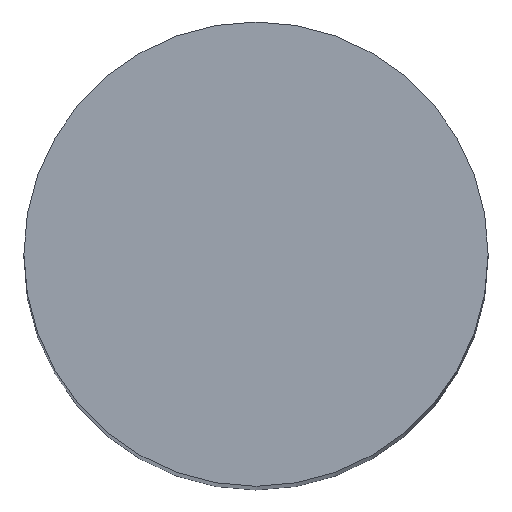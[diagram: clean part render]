
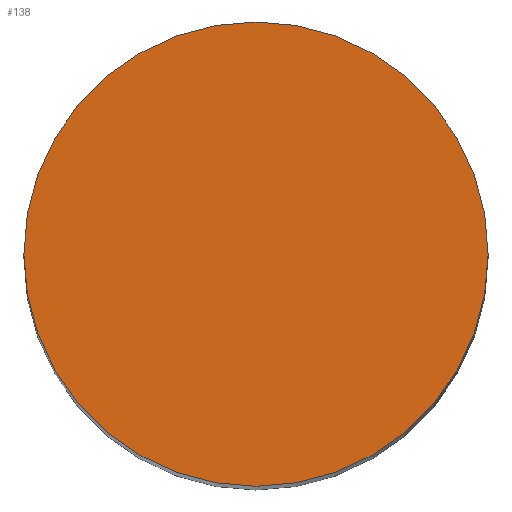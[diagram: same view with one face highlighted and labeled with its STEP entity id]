
A CAD part, top view. The second image highlights one B-rep face of the part: STEP entity #138.
In plain terms, the highlighted planar face has unit normal (0, 0, 1).
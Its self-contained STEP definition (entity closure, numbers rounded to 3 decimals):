
#3 = PLANE ( 'NONE',  #5 ) ;
#5 = AXIS2_PLACEMENT_3D ( 'NONE', #58, #28, #97 ) ;
#7 = CARTESIAN_POINT ( 'NONE',  ( 0., 0., 22.225 ) ) ;
#8 = EDGE_CURVE ( 'NONE', #111, #102, #110, .T. ) ;
#14 = DIRECTION ( 'NONE',  ( 0., 0., 1. ) ) ;
#27 = CARTESIAN_POINT ( 'NONE',  ( -2.413, 0., 22.225 ) ) ;
#28 = DIRECTION ( 'NONE',  ( 0., 0., 1. ) ) ;
#37 = FACE_OUTER_BOUND ( 'NONE', #47, .T. ) ;
#47 = EDGE_LOOP ( 'NONE', ( #103, #75 ) ) ;
#50 = CARTESIAN_POINT ( 'NONE',  ( 2.413, 0., 22.225 ) ) ;
#55 = DIRECTION ( 'NONE',  ( 1., 0., 0. ) ) ;
#58 = CARTESIAN_POINT ( 'NONE',  ( 0., 0., 22.225 ) ) ;
#68 = CARTESIAN_POINT ( 'NONE',  ( 0., 0., 22.225 ) ) ;
#75 = ORIENTED_EDGE ( 'NONE', *, *, #8, .T. ) ;
#80 = DIRECTION ( 'NONE',  ( 0., 0., 1. ) ) ;
#83 = AXIS2_PLACEMENT_3D ( 'NONE', #7, #14, #55 ) ;
#97 = DIRECTION ( 'NONE',  ( 1., 0., 0. ) ) ;
#99 = EDGE_CURVE ( 'NONE', #102, #111, #112, .T. ) ;
#102 = VERTEX_POINT ( 'NONE', #27 ) ;
#103 = ORIENTED_EDGE ( 'NONE', *, *, #99, .T. ) ;
#110 = CIRCLE ( 'NONE', #128, 2.413 ) ;
#111 = VERTEX_POINT ( 'NONE', #50 ) ;
#112 = CIRCLE ( 'NONE', #83, 2.413 ) ;
#115 = DIRECTION ( 'NONE',  ( 1., 0., 0. ) ) ;
#128 = AXIS2_PLACEMENT_3D ( 'NONE', #68, #80, #115 ) ;
#138 = ADVANCED_FACE ( 'NONE', ( #37 ), #3, .T. ) ;
